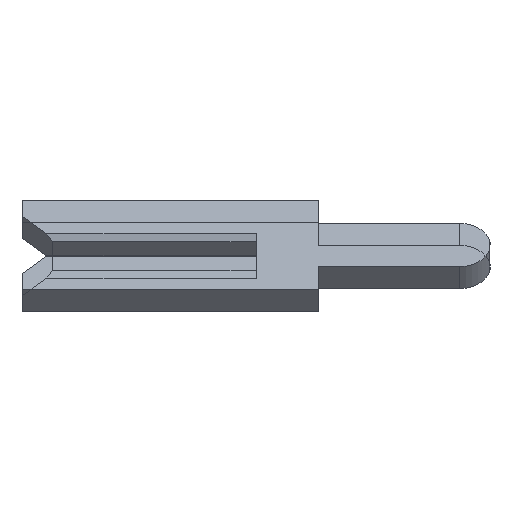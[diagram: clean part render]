
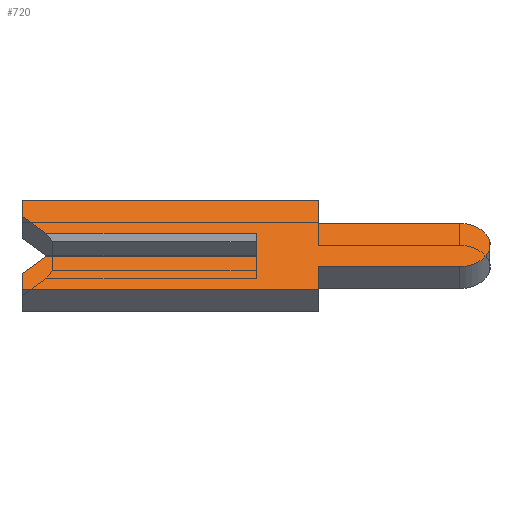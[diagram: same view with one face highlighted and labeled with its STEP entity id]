
A CAD part, left-side view. The second image highlights one B-rep face of the part: STEP entity #720.
In plain terms, the highlighted face is planar.
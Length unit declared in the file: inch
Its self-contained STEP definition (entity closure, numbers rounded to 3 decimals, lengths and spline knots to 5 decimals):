
#2 = ORIENTED_EDGE ( 'NONE', *, *, #3207, .F. ) ;
#15 = DIRECTION ( 'NONE',  ( 0., -1., 0. ) ) ;
#51 = VERTEX_POINT ( 'NONE', #3393 ) ;
#84 = DIRECTION ( 'NONE',  ( 0., 1., 0. ) ) ;
#125 = EDGE_CURVE ( 'NONE', #3874, #135, #2276, .T. ) ;
#135 = VERTEX_POINT ( 'NONE', #2137 ) ;
#139 = ORIENTED_EDGE ( 'NONE', *, *, #1138, .F. ) ;
#148 = LINE ( 'NONE', #1907, #558 ) ;
#157 = LINE ( 'NONE', #3464, #1059 ) ;
#187 = ORIENTED_EDGE ( 'NONE', *, *, #1413, .F. ) ;
#213 = VECTOR ( 'NONE', #2564, 39.37008 ) ;
#255 = LINE ( 'NONE', #3263, #1656 ) ;
#268 = VECTOR ( 'NONE', #507, 39.37008 ) ;
#269 = CARTESIAN_POINT ( 'NONE',  ( -0.01, 0.15, -0.04 ) ) ;
#283 = EDGE_CURVE ( 'NONE', #1275, #2754, #2181, .T. ) ;
#363 = LINE ( 'NONE', #1753, #1973 ) ;
#390 = ORIENTED_EDGE ( 'NONE', *, *, #3012, .F. ) ;
#394 = ORIENTED_EDGE ( 'NONE', *, *, #1708, .F. ) ;
#418 = LINE ( 'NONE', #669, #213 ) ;
#423 = AXIS2_PLACEMENT_3D ( 'NONE', #2846, #1885, #3526 ) ;
#470 = LINE ( 'NONE', #2073, #3290 ) ;
#474 = VECTOR ( 'NONE', #3766, 39.37008 ) ;
#507 = DIRECTION ( 'NONE',  ( 0., 0., -1. ) ) ;
#519 = VERTEX_POINT ( 'NONE', #3510 ) ;
#542 = DIRECTION ( 'NONE',  ( 0., 0., 1. ) ) ;
#558 = VECTOR ( 'NONE', #15, 39.37008 ) ;
#632 = CARTESIAN_POINT ( 'NONE',  ( -0.01, 0.15, 0.026 ) ) ;
#669 = CARTESIAN_POINT ( 'NONE',  ( -0.01, -0.04, -0.04 ) ) ;
#720 = ADVANCED_FACE ( 'NONE', ( #3605 ), #1250, .F. ) ;
#749 = CARTESIAN_POINT ( 'NONE',  ( -0.01, 0.15, 0.04 ) ) ;
#761 = LINE ( 'NONE', #2554, #1417 ) ;
#762 = ORIENTED_EDGE ( 'NONE', *, *, #125, .F. ) ;
#830 = CARTESIAN_POINT ( 'NONE',  ( -0.01, -0.04, 0.04 ) ) ;
#979 = EDGE_CURVE ( 'NONE', #4082, #1275, #157, .T. ) ;
#986 = DIRECTION ( 'NONE',  ( 0., 1., 0. ) ) ;
#999 = CARTESIAN_POINT ( 'NONE',  ( -0.01, -0.04, -0.0195 ) ) ;
#1055 = DIRECTION ( 'NONE',  ( 0., -1., 0. ) ) ;
#1059 = VECTOR ( 'NONE', #1513, 39.37008 ) ;
#1062 = VERTEX_POINT ( 'NONE', #269 ) ;
#1091 = ORIENTED_EDGE ( 'NONE', *, *, #2275, .F. ) ;
#1138 = EDGE_CURVE ( 'NONE', #3870, #1062, #1516, .T. ) ;
#1250 = PLANE ( 'NONE',  #423 ) ;
#1275 = VERTEX_POINT ( 'NONE', #632 ) ;
#1297 = CARTESIAN_POINT ( 'NONE',  ( -0.01, 0.15, -0.04 ) ) ;
#1319 = VECTOR ( 'NONE', #986, 39.37008 ) ;
#1413 = EDGE_CURVE ( 'NONE', #3241, #3870, #418, .T. ) ;
#1417 = VECTOR ( 'NONE', #3553, 39.37008 ) ;
#1453 = DIRECTION ( 'NONE',  ( 1., 0., 0. ) ) ;
#1513 = DIRECTION ( 'NONE',  ( 0., 0.707, 0.707 ) ) ;
#1516 = LINE ( 'NONE', #1297, #1319 ) ;
#1517 = ORIENTED_EDGE ( 'NONE', *, *, #4050, .F. ) ;
#1617 = ORIENTED_EDGE ( 'NONE', *, *, #1628, .F. ) ;
#1628 = EDGE_CURVE ( 'NONE', #135, #51, #761, .T. ) ;
#1656 = VECTOR ( 'NONE', #1055, 39.37008 ) ;
#1708 = EDGE_CURVE ( 'NONE', #519, #3088, #148, .T. ) ;
#1753 = CARTESIAN_POINT ( 'NONE',  ( -0.01, 0.1305, -0.0065 ) ) ;
#1854 = VERTEX_POINT ( 'NONE', #3315 ) ;
#1882 = AXIS2_PLACEMENT_3D ( 'NONE', #3681, #1453, #4013 ) ;
#1885 = DIRECTION ( 'NONE',  ( 1., 0., 0. ) ) ;
#1907 = CARTESIAN_POINT ( 'NONE',  ( -0.01, -0.1305, -0.01 ) ) ;
#1973 = VECTOR ( 'NONE', #3442, 39.37008 ) ;
#2061 = CARTESIAN_POINT ( 'NONE',  ( -0.01, -0.04, -0.0195 ) ) ;
#2073 = CARTESIAN_POINT ( 'NONE',  ( -0.01, 0.15, -0.026 ) ) ;
#2102 = CARTESIAN_POINT ( 'NONE',  ( -0.01, 0., 0.0065 ) ) ;
#2137 = CARTESIAN_POINT ( 'NONE',  ( -0.01, -0.04, 0.0195 ) ) ;
#2181 = LINE ( 'NONE', #2757, #474 ) ;
#2275 = EDGE_CURVE ( 'NONE', #4033, #3241, #4016, .T. ) ;
#2276 = LINE ( 'NONE', #2436, #268 ) ;
#2280 = EDGE_CURVE ( 'NONE', #4082, #1854, #255, .T. ) ;
#2370 = VECTOR ( 'NONE', #84, 39.37008 ) ;
#2431 = VERTEX_POINT ( 'NONE', #3279 ) ;
#2436 = CARTESIAN_POINT ( 'NONE',  ( -0.01, -0.04, 0.04 ) ) ;
#2459 = LINE ( 'NONE', #2102, #2612 ) ;
#2515 = ORIENTED_EDGE ( 'NONE', *, *, #2280, .T. ) ;
#2554 = CARTESIAN_POINT ( 'NONE',  ( -0.01, -0.04, 0.0195 ) ) ;
#2564 = DIRECTION ( 'NONE',  ( 0., 0., -1. ) ) ;
#2585 = ORIENTED_EDGE ( 'NONE', *, *, #3840, .F. ) ;
#2612 = VECTOR ( 'NONE', #542, 39.37008 ) ;
#2642 = ORIENTED_EDGE ( 'NONE', *, *, #283, .F. ) ;
#2718 = CARTESIAN_POINT ( 'NONE',  ( -0.01, 0., -0.01 ) ) ;
#2754 = VERTEX_POINT ( 'NONE', #749 ) ;
#2757 = CARTESIAN_POINT ( 'NONE',  ( -0.01, 0.15, 0.026 ) ) ;
#2803 = CIRCLE ( 'NONE', #1882, 0.0195 ) ;
#2846 = CARTESIAN_POINT ( 'NONE',  ( -0.01, -0.1305, 0. ) ) ;
#3012 = EDGE_CURVE ( 'NONE', #51, #4033, #2803, .T. ) ;
#3052 = VECTOR ( 'NONE', #3730, 39.37008 ) ;
#3088 = VERTEX_POINT ( 'NONE', #2718 ) ;
#3109 = CARTESIAN_POINT ( 'NONE',  ( -0.01, -0.1305, -0.0195 ) ) ;
#3123 = CARTESIAN_POINT ( 'NONE',  ( -0.01, 0.15, 0.04 ) ) ;
#3137 = CARTESIAN_POINT ( 'NONE',  ( -0.01, 0.134, 0.01 ) ) ;
#3193 = ORIENTED_EDGE ( 'NONE', *, *, #979, .F. ) ;
#3207 = EDGE_CURVE ( 'NONE', #1062, #2431, #470, .T. ) ;
#3241 = VERTEX_POINT ( 'NONE', #2061 ) ;
#3263 = CARTESIAN_POINT ( 'NONE',  ( -0.01, 0.15, 0.01 ) ) ;
#3279 = CARTESIAN_POINT ( 'NONE',  ( -0.01, 0.15, -0.026 ) ) ;
#3290 = VECTOR ( 'NONE', #4058, 39.37008 ) ;
#3294 = ORIENTED_EDGE ( 'NONE', *, *, #3397, .F. ) ;
#3315 = CARTESIAN_POINT ( 'NONE',  ( -0.01, 0., 0.01 ) ) ;
#3393 = CARTESIAN_POINT ( 'NONE',  ( -0.01, -0.1305, 0.0195 ) ) ;
#3397 = EDGE_CURVE ( 'NONE', #2431, #519, #363, .T. ) ;
#3442 = DIRECTION ( 'NONE',  ( 0., -0.707, 0.707 ) ) ;
#3464 = CARTESIAN_POINT ( 'NONE',  ( -0.01, 0.1305, 0.0065 ) ) ;
#3510 = CARTESIAN_POINT ( 'NONE',  ( -0.01, 0.134, -0.01 ) ) ;
#3526 = DIRECTION ( 'NONE',  ( 0., 0., -1. ) ) ;
#3553 = DIRECTION ( 'NONE',  ( 0., -1., 0. ) ) ;
#3605 = FACE_OUTER_BOUND ( 'NONE', #3896, .T. ) ;
#3616 = LINE ( 'NONE', #3123, #3052 ) ;
#3681 = CARTESIAN_POINT ( 'NONE',  ( -0.01, -0.1305, 0. ) ) ;
#3730 = DIRECTION ( 'NONE',  ( 0., -1., 0. ) ) ;
#3766 = DIRECTION ( 'NONE',  ( 0., 0., 1. ) ) ;
#3776 = CARTESIAN_POINT ( 'NONE',  ( -0.01, -0.04, -0.04 ) ) ;
#3840 = EDGE_CURVE ( 'NONE', #3088, #1854, #2459, .T. ) ;
#3870 = VERTEX_POINT ( 'NONE', #3776 ) ;
#3874 = VERTEX_POINT ( 'NONE', #830 ) ;
#3896 = EDGE_LOOP ( 'NONE', ( #2515, #2585, #394, #3294, #2, #139, #187, #1091, #390, #1617, #762, #1517, #2642, #3193 ) ) ;
#4013 = DIRECTION ( 'NONE',  ( 0., 0., -1. ) ) ;
#4016 = LINE ( 'NONE', #999, #2370 ) ;
#4033 = VERTEX_POINT ( 'NONE', #3109 ) ;
#4050 = EDGE_CURVE ( 'NONE', #2754, #3874, #3616, .T. ) ;
#4058 = DIRECTION ( 'NONE',  ( 0., 0., 1. ) ) ;
#4082 = VERTEX_POINT ( 'NONE', #3137 ) ;
